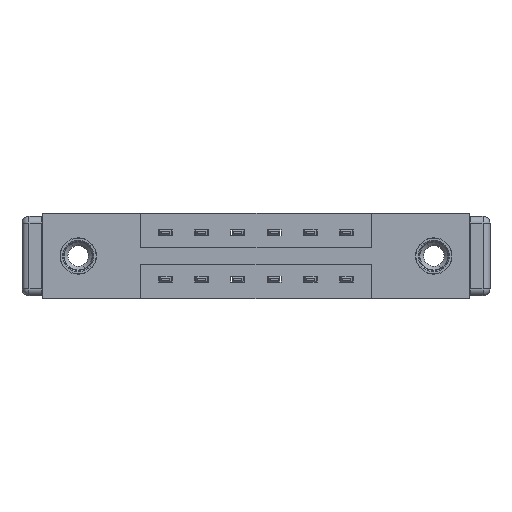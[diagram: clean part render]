
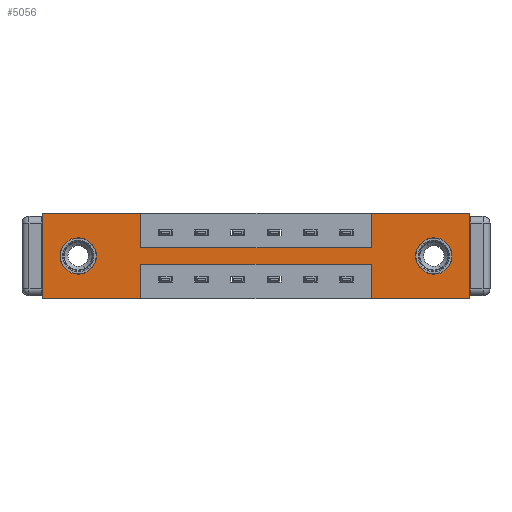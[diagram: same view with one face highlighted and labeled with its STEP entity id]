
A CAD part, front view. The second image highlights one B-rep face of the part: STEP entity #5056.
In plain terms, the highlighted planar face has unit normal (0, -1, 0).
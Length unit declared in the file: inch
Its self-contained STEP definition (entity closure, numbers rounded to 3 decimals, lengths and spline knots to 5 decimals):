
#10 = EDGE_CURVE ( 'NONE', #1940, #5010, #2548, .T. ) ;
#152 = EDGE_CURVE ( 'NONE', #3319, #6709, #10443, .T. ) ;
#237 = VERTEX_POINT ( 'NONE', #3906 ) ;
#251 = LINE ( 'NONE', #611, #391 ) ;
#330 = DIRECTION ( 'NONE',  ( 0., 0., -1. ) ) ;
#391 = VECTOR ( 'NONE', #4297, 39.37008 ) ;
#611 = CARTESIAN_POINT ( 'NONE',  ( 0., 0., 0. ) ) ;
#653 = EDGE_CURVE ( 'NONE', #8094, #5760, #5957, .T. ) ;
#745 = DIRECTION ( 'NONE',  ( 0., 0., -1. ) ) ;
#900 = CARTESIAN_POINT ( 'NONE',  ( 0.155, 0., -0.185 ) ) ;
#905 = LINE ( 'NONE', #4409, #11088 ) ;
#1028 = EDGE_LOOP ( 'NONE', ( #3011, #1052 ) ) ;
#1052 = ORIENTED_EDGE ( 'NONE', *, *, #152, .T. ) ;
#1159 = CARTESIAN_POINT ( 'NONE',  ( 1.687, 0., -0.263 ) ) ;
#1211 = EDGE_CURVE ( 'NONE', #6709, #3319, #10991, .T. ) ;
#1395 = EDGE_CURVE ( 'NONE', #3112, #8426, #11816, .T. ) ;
#1493 = CARTESIAN_POINT ( 'NONE',  ( 0., 0., -0.37 ) ) ;
#1591 = DIRECTION ( 'NONE',  ( 0., 0., -1. ) ) ;
#1601 = CARTESIAN_POINT ( 'NONE',  ( 1.417, 0., -0.37 ) ) ;
#1681 = CARTESIAN_POINT ( 'NONE',  ( 0.425, 0., -0.37 ) ) ;
#1764 = ORIENTED_EDGE ( 'NONE', *, *, #1395, .F. ) ;
#1917 = CARTESIAN_POINT ( 'NONE',  ( 0., 0., 0. ) ) ;
#1925 = CARTESIAN_POINT ( 'NONE',  ( 1.842, 0., 0. ) ) ;
#1940 = VERTEX_POINT ( 'NONE', #4554 ) ;
#2020 = FACE_BOUND ( 'NONE', #1028, .T. ) ;
#2071 = VECTOR ( 'NONE', #2913, 39.37008 ) ;
#2099 = DIRECTION ( 'NONE',  ( 0., 1., 0. ) ) ;
#2272 = ORIENTED_EDGE ( 'NONE', *, *, #10, .F. ) ;
#2354 = EDGE_CURVE ( 'NONE', #4636, #3649, #905, .T. ) ;
#2379 = VECTOR ( 'NONE', #330, 39.37008 ) ;
#2548 = LINE ( 'NONE', #8504, #8985 ) ;
#2634 = EDGE_CURVE ( 'NONE', #11911, #7448, #8381, .T. ) ;
#2650 = CARTESIAN_POINT ( 'NONE',  ( 0.155, 0., -0.263 ) ) ;
#2837 = DIRECTION ( 'NONE',  ( 0., 0., 1. ) ) ;
#2885 = ORIENTED_EDGE ( 'NONE', *, *, #8420, .F. ) ;
#2913 = DIRECTION ( 'NONE',  ( 0., 0., -1. ) ) ;
#2952 = EDGE_CURVE ( 'NONE', #237, #1940, #8367, .T. ) ;
#2986 = CARTESIAN_POINT ( 'NONE',  ( 1.417, 0., -0.22 ) ) ;
#3011 = ORIENTED_EDGE ( 'NONE', *, *, #1211, .T. ) ;
#3045 = DIRECTION ( 'NONE',  ( 0., 0., -1. ) ) ;
#3112 = VERTEX_POINT ( 'NONE', #3121 ) ;
#3121 = CARTESIAN_POINT ( 'NONE',  ( 0.425, 0., 0. ) ) ;
#3319 = VERTEX_POINT ( 'NONE', #2650 ) ;
#3403 = CARTESIAN_POINT ( 'NONE',  ( 1.417, 0., -0.37 ) ) ;
#3421 = LINE ( 'NONE', #10508, #6541 ) ;
#3556 = VECTOR ( 'NONE', #3772, 39.37008 ) ;
#3583 = CARTESIAN_POINT ( 'NONE',  ( 1.687, 0., -0.185 ) ) ;
#3649 = VERTEX_POINT ( 'NONE', #6521 ) ;
#3772 = DIRECTION ( 'NONE',  ( -1., 0., 0. ) ) ;
#3806 = CARTESIAN_POINT ( 'NONE',  ( 1.417, 0., -0.15 ) ) ;
#3906 = CARTESIAN_POINT ( 'NONE',  ( 1.842, 0., 0. ) ) ;
#4015 = LINE ( 'NONE', #6314, #6878 ) ;
#4188 = ORIENTED_EDGE ( 'NONE', *, *, #2952, .F. ) ;
#4297 = DIRECTION ( 'NONE',  ( 1., 0., 0. ) ) ;
#4409 = CARTESIAN_POINT ( 'NONE',  ( 1.417, 0., 0. ) ) ;
#4414 = VECTOR ( 'NONE', #745, 39.37008 ) ;
#4456 = CARTESIAN_POINT ( 'NONE',  ( 1.687, 0., -0.107 ) ) ;
#4479 = ORIENTED_EDGE ( 'NONE', *, *, #8261, .F. ) ;
#4499 = DIRECTION ( 'NONE',  ( 0., 0., 1. ) ) ;
#4522 = EDGE_CURVE ( 'NONE', #3649, #237, #4015, .T. ) ;
#4541 = LINE ( 'NONE', #8353, #3556 ) ;
#4554 = CARTESIAN_POINT ( 'NONE',  ( 1.842, 0., -0.37 ) ) ;
#4636 = VERTEX_POINT ( 'NONE', #3806 ) ;
#4742 = CARTESIAN_POINT ( 'NONE',  ( 0.155, 0., -0.107 ) ) ;
#5010 = VERTEX_POINT ( 'NONE', #3403 ) ;
#5056 = ADVANCED_FACE ( 'NONE', ( #9612, #2020, #10769 ), #9979, .T. ) ;
#5066 = CARTESIAN_POINT ( 'NONE',  ( 0.425, 0., 0. ) ) ;
#5351 = VECTOR ( 'NONE', #2837, 39.37008 ) ;
#5356 = VERTEX_POINT ( 'NONE', #6662 ) ;
#5551 = CARTESIAN_POINT ( 'NONE',  ( 0.425, 0., -0.22 ) ) ;
#5556 = EDGE_CURVE ( 'NONE', #7448, #3112, #251, .T. ) ;
#5754 = ORIENTED_EDGE ( 'NONE', *, *, #4522, .F. ) ;
#5760 = VERTEX_POINT ( 'NONE', #4456 ) ;
#5858 = EDGE_CURVE ( 'NONE', #5356, #11911, #4541, .T. ) ;
#5903 = CARTESIAN_POINT ( 'NONE',  ( 0.425, 0., -0.22 ) ) ;
#5951 = ORIENTED_EDGE ( 'NONE', *, *, #11151, .T. ) ;
#5957 = CIRCLE ( 'NONE', #11411, 0.078 ) ;
#6047 = DIRECTION ( 'NONE',  ( 1., 0., 0. ) ) ;
#6097 = EDGE_LOOP ( 'NONE', ( #5951, #6854 ) ) ;
#6248 = DIRECTION ( 'NONE',  ( 0., 1., 0. ) ) ;
#6314 = CARTESIAN_POINT ( 'NONE',  ( 0., 0., 0. ) ) ;
#6321 = AXIS2_PLACEMENT_3D ( 'NONE', #900, #8243, #10171 ) ;
#6432 = AXIS2_PLACEMENT_3D ( 'NONE', #3583, #6248, #1591 ) ;
#6521 = CARTESIAN_POINT ( 'NONE',  ( 1.417, 0., 0. ) ) ;
#6541 = VECTOR ( 'NONE', #6047, 39.37008 ) ;
#6662 = CARTESIAN_POINT ( 'NONE',  ( 0.425, 0., -0.37 ) ) ;
#6665 = EDGE_CURVE ( 'NONE', #8594, #8148, #8418, .T. ) ;
#6709 = VERTEX_POINT ( 'NONE', #4742 ) ;
#6854 = ORIENTED_EDGE ( 'NONE', *, *, #653, .T. ) ;
#6878 = VECTOR ( 'NONE', #9180, 39.37008 ) ;
#6886 = EDGE_LOOP ( 'NONE', ( #4479, #7495, #2885, #2272, #4188, #5754, #9808, #8359, #1764, #10460, #7603, #8313 ) ) ;
#7098 = CARTESIAN_POINT ( 'NONE',  ( 0.425, 0., -0.15 ) ) ;
#7354 = CIRCLE ( 'NONE', #6432, 0.078 ) ;
#7448 = VERTEX_POINT ( 'NONE', #10274 ) ;
#7495 = ORIENTED_EDGE ( 'NONE', *, *, #6665, .F. ) ;
#7555 = CARTESIAN_POINT ( 'NONE',  ( 1.687, 0., -0.185 ) ) ;
#7573 = DIRECTION ( 'NONE',  ( 0., 0., 1. ) ) ;
#7603 = ORIENTED_EDGE ( 'NONE', *, *, #2634, .F. ) ;
#7839 = VECTOR ( 'NONE', #4499, 39.37008 ) ;
#8094 = VERTEX_POINT ( 'NONE', #1159 ) ;
#8148 = VERTEX_POINT ( 'NONE', #5903 ) ;
#8241 = EDGE_CURVE ( 'NONE', #8426, #4636, #3421, .T. ) ;
#8243 = DIRECTION ( 'NONE',  ( 0., 1., 0. ) ) ;
#8261 = EDGE_CURVE ( 'NONE', #8148, #5356, #10742, .T. ) ;
#8313 = ORIENTED_EDGE ( 'NONE', *, *, #5858, .F. ) ;
#8353 = CARTESIAN_POINT ( 'NONE',  ( 0., 0., -0.37 ) ) ;
#8359 = ORIENTED_EDGE ( 'NONE', *, *, #8241, .F. ) ;
#8367 = LINE ( 'NONE', #1925, #2071 ) ;
#8381 = LINE ( 'NONE', #1917, #5351 ) ;
#8418 = LINE ( 'NONE', #5551, #9275 ) ;
#8420 = EDGE_CURVE ( 'NONE', #5010, #8594, #10296, .T. ) ;
#8426 = VERTEX_POINT ( 'NONE', #7098 ) ;
#8479 = AXIS2_PLACEMENT_3D ( 'NONE', #10822, #9005, #11636 ) ;
#8492 = CARTESIAN_POINT ( 'NONE',  ( 0.155, 0., -0.185 ) ) ;
#8504 = CARTESIAN_POINT ( 'NONE',  ( 0., 0., -0.37 ) ) ;
#8594 = VERTEX_POINT ( 'NONE', #2986 ) ;
#8612 = DIRECTION ( 'NONE',  ( -1., 0., 0. ) ) ;
#8985 = VECTOR ( 'NONE', #8612, 39.37008 ) ;
#9005 = DIRECTION ( 'NONE',  ( 0., -1., 0. ) ) ;
#9180 = DIRECTION ( 'NONE',  ( 1., 0., 0. ) ) ;
#9275 = VECTOR ( 'NONE', #9375, 39.37008 ) ;
#9325 = DIRECTION ( 'NONE',  ( 0., 1., 0. ) ) ;
#9346 = AXIS2_PLACEMENT_3D ( 'NONE', #8492, #9325, #7573 ) ;
#9375 = DIRECTION ( 'NONE',  ( -1., 0., 0. ) ) ;
#9612 = FACE_BOUND ( 'NONE', #6097, .T. ) ;
#9808 = ORIENTED_EDGE ( 'NONE', *, *, #2354, .F. ) ;
#9979 = PLANE ( 'NONE',  #8479 ) ;
#10171 = DIRECTION ( 'NONE',  ( 0., 0., 1. ) ) ;
#10274 = CARTESIAN_POINT ( 'NONE',  ( 0., 0., 0. ) ) ;
#10296 = LINE ( 'NONE', #1601, #7839 ) ;
#10443 = CIRCLE ( 'NONE', #6321, 0.078 ) ;
#10460 = ORIENTED_EDGE ( 'NONE', *, *, #5556, .F. ) ;
#10508 = CARTESIAN_POINT ( 'NONE',  ( 0.425, 0., -0.15 ) ) ;
#10742 = LINE ( 'NONE', #1681, #4414 ) ;
#10769 = FACE_OUTER_BOUND ( 'NONE', #6886, .T. ) ;
#10822 = CARTESIAN_POINT ( 'NONE',  ( 0., 0., -0.37 ) ) ;
#10991 = CIRCLE ( 'NONE', #9346, 0.078 ) ;
#11088 = VECTOR ( 'NONE', #11817, 39.37008 ) ;
#11151 = EDGE_CURVE ( 'NONE', #5760, #8094, #7354, .T. ) ;
#11411 = AXIS2_PLACEMENT_3D ( 'NONE', #7555, #2099, #3045 ) ;
#11636 = DIRECTION ( 'NONE',  ( 0., 0., -1. ) ) ;
#11816 = LINE ( 'NONE', #5066, #2379 ) ;
#11817 = DIRECTION ( 'NONE',  ( 0., 0., 1. ) ) ;
#11911 = VERTEX_POINT ( 'NONE', #1493 ) ;
